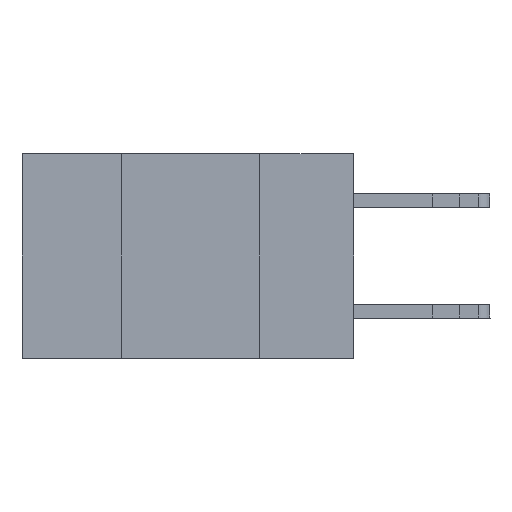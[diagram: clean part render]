
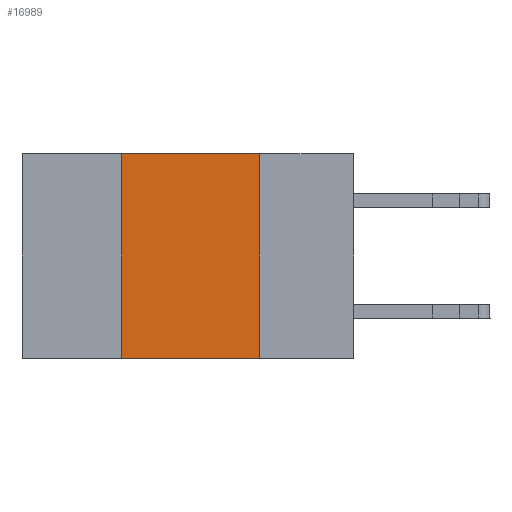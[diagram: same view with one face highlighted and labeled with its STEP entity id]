
A CAD part, left-side view. The second image highlights one B-rep face of the part: STEP entity #16989.
In plain terms, the highlighted planar face has unit normal (-1, 0, 0).
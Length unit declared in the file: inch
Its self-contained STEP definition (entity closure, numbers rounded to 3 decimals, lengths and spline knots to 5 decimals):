
#1208 = VECTOR ( 'NONE', #25289, 39.37008 ) ;
#1295 = ORIENTED_EDGE ( 'NONE', *, *, #22921, .F. ) ;
#1495 = VERTEX_POINT ( 'NONE', #29055 ) ;
#5482 = VECTOR ( 'NONE', #18239, 39.37008 ) ;
#6112 = LINE ( 'NONE', #29791, #5482 ) ;
#6485 = DIRECTION ( 'NONE',  ( 0., -1., 0. ) ) ;
#6568 = DIRECTION ( 'NONE',  ( 0., 0., -1. ) ) ;
#7211 = LINE ( 'NONE', #32634, #36948 ) ;
#8304 = CARTESIAN_POINT ( 'NONE',  ( 0., 0.42, -0.37 ) ) ;
#9253 = CARTESIAN_POINT ( 'NONE',  ( 0., 0.17, -0.37 ) ) ;
#9649 = FACE_OUTER_BOUND ( 'NONE', #22184, .T. ) ;
#10243 = CARTESIAN_POINT ( 'NONE',  ( 0., 0.6, 0. ) ) ;
#12408 = VECTOR ( 'NONE', #24483, 39.37008 ) ;
#12946 = LINE ( 'NONE', #19115, #12408 ) ;
#13034 = VERTEX_POINT ( 'NONE', #9253 ) ;
#14126 = VERTEX_POINT ( 'NONE', #26212 ) ;
#14556 = ORIENTED_EDGE ( 'NONE', *, *, #33249, .F. ) ;
#16831 = LINE ( 'NONE', #31252, #1208 ) ;
#16989 = ADVANCED_FACE ( 'NONE', ( #9649 ), #21368, .F. ) ;
#18239 = DIRECTION ( 'NONE',  ( 0., 0., 1. ) ) ;
#19115 = CARTESIAN_POINT ( 'NONE',  ( 0., 0.6, -0.37 ) ) ;
#19298 = ORIENTED_EDGE ( 'NONE', *, *, #36788, .T. ) ;
#20744 = AXIS2_PLACEMENT_3D ( 'NONE', #10243, #21948, #6568 ) ;
#21368 = PLANE ( 'NONE',  #20744 ) ;
#21948 = DIRECTION ( 'NONE',  ( 1., 0., 0. ) ) ;
#22184 = EDGE_LOOP ( 'NONE', ( #28308, #1295, #14556, #19298 ) ) ;
#22921 = EDGE_CURVE ( 'NONE', #1495, #14126, #7211, .T. ) ;
#24483 = DIRECTION ( 'NONE',  ( 0., -1., 0. ) ) ;
#25289 = DIRECTION ( 'NONE',  ( 0., 0., -1. ) ) ;
#26212 = CARTESIAN_POINT ( 'NONE',  ( 0., 0.17, 0. ) ) ;
#28308 = ORIENTED_EDGE ( 'NONE', *, *, #33894, .F. ) ;
#28325 = VERTEX_POINT ( 'NONE', #8304 ) ;
#29055 = CARTESIAN_POINT ( 'NONE',  ( 0., 0.42, 0. ) ) ;
#29791 = CARTESIAN_POINT ( 'NONE',  ( 0., 0.42, 0. ) ) ;
#31252 = CARTESIAN_POINT ( 'NONE',  ( 0., 0.17, 0. ) ) ;
#32634 = CARTESIAN_POINT ( 'NONE',  ( 0., 0.6, 0. ) ) ;
#33249 = EDGE_CURVE ( 'NONE', #28325, #1495, #6112, .T. ) ;
#33894 = EDGE_CURVE ( 'NONE', #14126, #13034, #16831, .T. ) ;
#36788 = EDGE_CURVE ( 'NONE', #28325, #13034, #12946, .T. ) ;
#36948 = VECTOR ( 'NONE', #6485, 39.37008 ) ;
